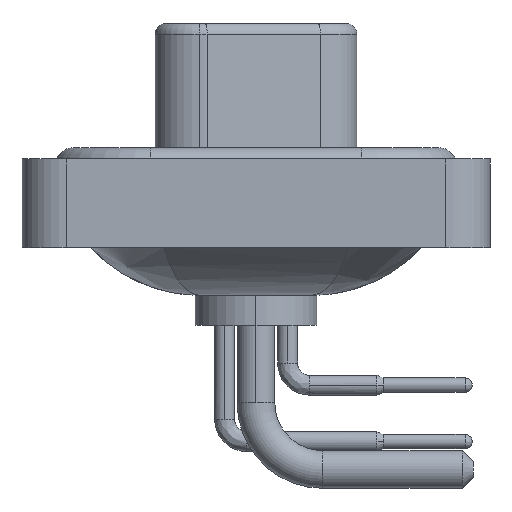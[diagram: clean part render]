
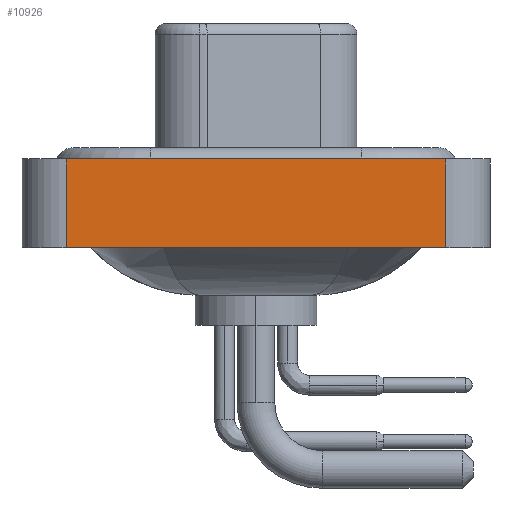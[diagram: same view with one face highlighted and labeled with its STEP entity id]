
A CAD part, left-side view. The second image highlights one B-rep face of the part: STEP entity #10926.
In plain terms, the highlighted planar face has unit normal (-1, 0, 0).
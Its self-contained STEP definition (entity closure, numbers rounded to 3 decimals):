
#754 = EDGE_CURVE ( 'NONE', #14974, #9250, #3285, .T. ) ;
#1513 = VECTOR ( 'NONE', #18986, 1000. ) ;
#2307 = CARTESIAN_POINT ( 'NONE',  ( -7.3, -8.55, -3.6 ) ) ;
#3285 = LINE ( 'NONE', #14480, #21696 ) ;
#3391 = CARTESIAN_POINT ( 'NONE',  ( -7.3, 8.55, -3.6 ) ) ;
#3624 = ORIENTED_EDGE ( 'NONE', *, *, #6386, .T. ) ;
#3811 = LINE ( 'NONE', #23096, #1513 ) ;
#4297 = DIRECTION ( 'NONE',  ( 0., 0., 1. ) ) ;
#4473 = CARTESIAN_POINT ( 'NONE',  ( -7.3, -8.55, -3.6 ) ) ;
#5196 = DIRECTION ( 'NONE',  ( -1., 0., 0. ) ) ;
#5409 = DIRECTION ( 'NONE',  ( 0., -1., 0. ) ) ;
#6386 = EDGE_CURVE ( 'NONE', #15674, #15274, #11788, .T. ) ;
#6406 = CARTESIAN_POINT ( 'NONE',  ( -7.3, 8.55, 0.4 ) ) ;
#7083 = CARTESIAN_POINT ( 'NONE',  ( -7.3, -8.55, -3.6 ) ) ;
#7419 = DIRECTION ( 'NONE',  ( 0., 0., 1. ) ) ;
#9250 = VERTEX_POINT ( 'NONE', #6406 ) ;
#9749 = CARTESIAN_POINT ( 'NONE',  ( -7.3, -8.55, 0.4 ) ) ;
#10926 = ADVANCED_FACE ( 'NONE', ( #18375 ), #24121, .T. ) ;
#11788 = LINE ( 'NONE', #2307, #15212 ) ;
#14480 = CARTESIAN_POINT ( 'NONE',  ( -7.3, 8.55, -3.6 ) ) ;
#14974 = VERTEX_POINT ( 'NONE', #3391 ) ;
#15212 = VECTOR ( 'NONE', #4297, 1000. ) ;
#15274 = VERTEX_POINT ( 'NONE', #9749 ) ;
#15674 = VERTEX_POINT ( 'NONE', #4473 ) ;
#16621 = DIRECTION ( 'NONE',  ( 0., 0., 1. ) ) ;
#16638 = VECTOR ( 'NONE', #5409, 1000. ) ;
#17748 = AXIS2_PLACEMENT_3D ( 'NONE', #7083, #5196, #16621 ) ;
#18143 = ORIENTED_EDGE ( 'NONE', *, *, #20872, .F. ) ;
#18330 = ORIENTED_EDGE ( 'NONE', *, *, #21371, .T. ) ;
#18375 = FACE_OUTER_BOUND ( 'NONE', #18430, .T. ) ;
#18430 = EDGE_LOOP ( 'NONE', ( #3624, #18143, #19070, #18330 ) ) ;
#18711 = CARTESIAN_POINT ( 'NONE',  ( -7.3, -8.55, -3.6 ) ) ;
#18955 = LINE ( 'NONE', #18711, #16638 ) ;
#18986 = DIRECTION ( 'NONE',  ( 0., -1., 0. ) ) ;
#19070 = ORIENTED_EDGE ( 'NONE', *, *, #754, .F. ) ;
#20872 = EDGE_CURVE ( 'NONE', #9250, #15274, #3811, .T. ) ;
#21371 = EDGE_CURVE ( 'NONE', #14974, #15674, #18955, .T. ) ;
#21696 = VECTOR ( 'NONE', #7419, 1000. ) ;
#23096 = CARTESIAN_POINT ( 'NONE',  ( -7.3, -8.55, 0.4 ) ) ;
#24121 = PLANE ( 'NONE',  #17748 ) ;
